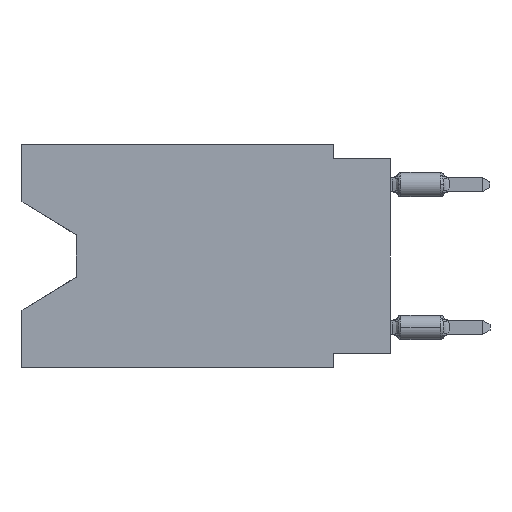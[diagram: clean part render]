
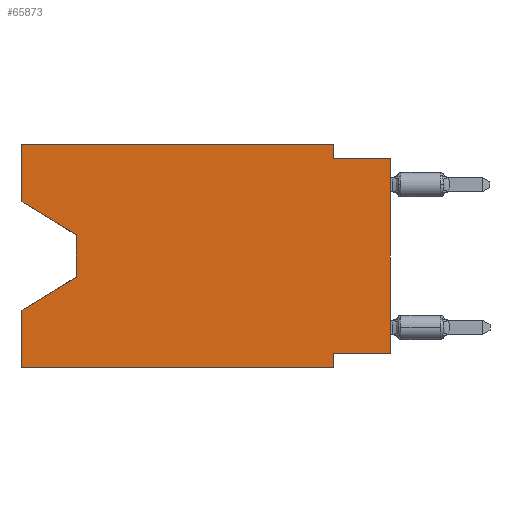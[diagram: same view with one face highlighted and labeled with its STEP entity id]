
A CAD part, left-side view. The second image highlights one B-rep face of the part: STEP entity #65873.
In plain terms, the highlighted planar face has unit normal (-1, 0, 0).
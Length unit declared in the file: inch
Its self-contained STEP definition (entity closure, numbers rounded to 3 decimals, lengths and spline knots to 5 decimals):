
#1302 = VECTOR ( 'NONE', #42875, 39.37008 ) ;
#1344 = CARTESIAN_POINT ( 'NONE',  ( 0., 0.645, -0.10025 ) ) ;
#1476 = CARTESIAN_POINT ( 'NONE',  ( 0., 0., -0.025 ) ) ;
#1651 = ORIENTED_EDGE ( 'NONE', *, *, #16922, .F. ) ;
#2779 = VERTEX_POINT ( 'NONE', #46725 ) ;
#2797 = ORIENTED_EDGE ( 'NONE', *, *, #29867, .F. ) ;
#3014 = VECTOR ( 'NONE', #8426, 39.37008 ) ;
#5950 = DIRECTION ( 'NONE',  ( 0., 0.855, -0.519 ) ) ;
#6667 = LINE ( 'NONE', #6993, #1302 ) ;
#6868 = VERTEX_POINT ( 'NONE', #1344 ) ;
#6993 = CARTESIAN_POINT ( 'NONE',  ( 0., 0.645, 0. ) ) ;
#8360 = EDGE_CURVE ( 'NONE', #6868, #58544, #62294, .T. ) ;
#8426 = DIRECTION ( 'NONE',  ( 0., 1., 0. ) ) ;
#9888 = ORIENTED_EDGE ( 'NONE', *, *, #42472, .T. ) ;
#12439 = LINE ( 'NONE', #23157, #60072 ) ;
#12981 = VERTEX_POINT ( 'NONE', #29851 ) ;
#13698 = VECTOR ( 'NONE', #49437, 39.37008 ) ;
#15011 = CARTESIAN_POINT ( 'NONE',  ( 0., 0.55, -0.158 ) ) ;
#15320 = LINE ( 'NONE', #41799, #58562 ) ;
#16042 = CARTESIAN_POINT ( 'NONE',  ( 0., 0.645, 0. ) ) ;
#16366 = CARTESIAN_POINT ( 'NONE',  ( 0., 0.645, 0. ) ) ;
#16922 = EDGE_CURVE ( 'NONE', #31438, #51498, #6667, .T. ) ;
#17970 = VERTEX_POINT ( 'NONE', #65999 ) ;
#18145 = DIRECTION ( 'NONE',  ( 0., 0., -1. ) ) ;
#18169 = CARTESIAN_POINT ( 'NONE',  ( 0., 0.1, 0. ) ) ;
#18789 = VERTEX_POINT ( 'NONE', #1476 ) ;
#19685 = LINE ( 'NONE', #15011, #43833 ) ;
#20385 = DIRECTION ( 'NONE',  ( 0., -0.855, -0.519 ) ) ;
#20720 = LINE ( 'NONE', #16042, #49266 ) ;
#20943 = CARTESIAN_POINT ( 'NONE',  ( 0., 0., -0.025 ) ) ;
#21895 = ORIENTED_EDGE ( 'NONE', *, *, #64167, .F. ) ;
#23157 = CARTESIAN_POINT ( 'NONE',  ( 0., 0.1, -0.39 ) ) ;
#23529 = CARTESIAN_POINT ( 'NONE',  ( 0., 0., -0.365 ) ) ;
#24148 = VERTEX_POINT ( 'NONE', #57727 ) ;
#25071 = CARTESIAN_POINT ( 'NONE',  ( 0., 0.645, -0.10025 ) ) ;
#25599 = VERTEX_POINT ( 'NONE', #18169 ) ;
#26421 = DIRECTION ( 'NONE',  ( 1., 0., 0. ) ) ;
#26831 = EDGE_CURVE ( 'NONE', #55057, #17970, #39901, .T. ) ;
#27643 = EDGE_CURVE ( 'NONE', #24148, #51498, #43151, .T. ) ;
#27730 = LINE ( 'NONE', #55739, #65139 ) ;
#28014 = CARTESIAN_POINT ( 'NONE',  ( 0., 0.645, 0. ) ) ;
#29851 = CARTESIAN_POINT ( 'NONE',  ( 0., 0.1, -0.39 ) ) ;
#29867 = EDGE_CURVE ( 'NONE', #17970, #12981, #12439, .T. ) ;
#31438 = VERTEX_POINT ( 'NONE', #46915 ) ;
#31736 = CARTESIAN_POINT ( 'NONE',  ( 0., 0.1, -0.025 ) ) ;
#33389 = AXIS2_PLACEMENT_3D ( 'NONE', #28014, #26421, #53132 ) ;
#35808 = ORIENTED_EDGE ( 'NONE', *, *, #61640, .T. ) ;
#35923 = CARTESIAN_POINT ( 'NONE',  ( 0., 0., -0.365 ) ) ;
#36287 = VECTOR ( 'NONE', #5950, 39.37008 ) ;
#36487 = DIRECTION ( 'NONE',  ( 0., -1., 0. ) ) ;
#39202 = VECTOR ( 'NONE', #40835, 39.37008 ) ;
#39901 = LINE ( 'NONE', #23529, #3014 ) ;
#40132 = DIRECTION ( 'NONE',  ( 0., 0., -1. ) ) ;
#40732 = DIRECTION ( 'NONE',  ( 0., -1., 0. ) ) ;
#40835 = DIRECTION ( 'NONE',  ( 0., 0., 1. ) ) ;
#40874 = CARTESIAN_POINT ( 'NONE',  ( 0., 0.645, 0. ) ) ;
#41799 = CARTESIAN_POINT ( 'NONE',  ( 0., 0.1, 0. ) ) ;
#41889 = EDGE_LOOP ( 'NONE', ( #35808, #9888, #44199, #1651, #50164, #2797, #48529, #51282, #57090, #54850, #21895, #52132 ) ) ;
#42277 = VECTOR ( 'NONE', #40732, 39.37008 ) ;
#42472 = EDGE_CURVE ( 'NONE', #2779, #24148, #19685, .T. ) ;
#42875 = DIRECTION ( 'NONE',  ( 0., 0., 1. ) ) ;
#43022 = EDGE_CURVE ( 'NONE', #50867, #18789, #51115, .T. ) ;
#43151 = LINE ( 'NONE', #58574, #36287 ) ;
#43833 = VECTOR ( 'NONE', #40132, 39.37008 ) ;
#44199 = ORIENTED_EDGE ( 'NONE', *, *, #27643, .T. ) ;
#44391 = CARTESIAN_POINT ( 'NONE',  ( 0., 0., 0. ) ) ;
#45892 = EDGE_CURVE ( 'NONE', #25599, #50867, #15320, .T. ) ;
#46725 = CARTESIAN_POINT ( 'NONE',  ( 0., 0.55, -0.158 ) ) ;
#46915 = CARTESIAN_POINT ( 'NONE',  ( 0., 0.645, -0.39 ) ) ;
#48529 = ORIENTED_EDGE ( 'NONE', *, *, #26831, .F. ) ;
#48541 = EDGE_CURVE ( 'NONE', #55057, #18789, #58862, .T. ) ;
#49266 = VECTOR ( 'NONE', #36487, 39.37008 ) ;
#49437 = DIRECTION ( 'NONE',  ( 0., 0., 1. ) ) ;
#50164 = ORIENTED_EDGE ( 'NONE', *, *, #62040, .T. ) ;
#50867 = VERTEX_POINT ( 'NONE', #31736 ) ;
#51067 = CARTESIAN_POINT ( 'NONE',  ( 0., 0.645, -0.28975 ) ) ;
#51115 = LINE ( 'NONE', #20943, #42277 ) ;
#51236 = PLANE ( 'NONE',  #33389 ) ;
#51282 = ORIENTED_EDGE ( 'NONE', *, *, #48541, .T. ) ;
#51498 = VERTEX_POINT ( 'NONE', #51067 ) ;
#52132 = ORIENTED_EDGE ( 'NONE', *, *, #8360, .F. ) ;
#53132 = DIRECTION ( 'NONE',  ( 0., 0., -1. ) ) ;
#54850 = ORIENTED_EDGE ( 'NONE', *, *, #45892, .F. ) ;
#55057 = VERTEX_POINT ( 'NONE', #35923 ) ;
#55739 = CARTESIAN_POINT ( 'NONE',  ( 0., 0.645, -0.39 ) ) ;
#57090 = ORIENTED_EDGE ( 'NONE', *, *, #43022, .F. ) ;
#57212 = DIRECTION ( 'NONE',  ( 0., 0., -1. ) ) ;
#57727 = CARTESIAN_POINT ( 'NONE',  ( 0., 0.55, -0.232 ) ) ;
#58544 = VERTEX_POINT ( 'NONE', #40874 ) ;
#58562 = VECTOR ( 'NONE', #57212, 39.37008 ) ;
#58574 = CARTESIAN_POINT ( 'NONE',  ( 0., 0.55, -0.232 ) ) ;
#58862 = LINE ( 'NONE', #44391, #13698 ) ;
#60072 = VECTOR ( 'NONE', #18145, 39.37008 ) ;
#61632 = FACE_OUTER_BOUND ( 'NONE', #41889, .T. ) ;
#61640 = EDGE_CURVE ( 'NONE', #6868, #2779, #65940, .T. ) ;
#62040 = EDGE_CURVE ( 'NONE', #31438, #12981, #27730, .T. ) ;
#62294 = LINE ( 'NONE', #16366, #39202 ) ;
#64167 = EDGE_CURVE ( 'NONE', #58544, #25599, #20720, .T. ) ;
#64258 = DIRECTION ( 'NONE',  ( 0., -1., 0. ) ) ;
#65139 = VECTOR ( 'NONE', #64258, 39.37008 ) ;
#65239 = VECTOR ( 'NONE', #20385, 39.37008 ) ;
#65873 = ADVANCED_FACE ( 'NONE', ( #61632 ), #51236, .F. ) ;
#65940 = LINE ( 'NONE', #25071, #65239 ) ;
#65999 = CARTESIAN_POINT ( 'NONE',  ( 0., 0.1, -0.365 ) ) ;
